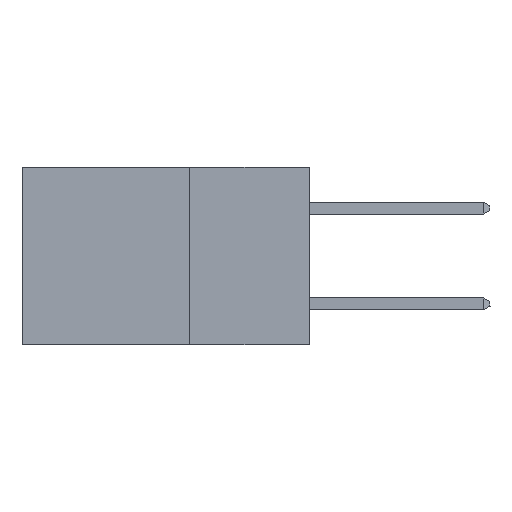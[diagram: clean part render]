
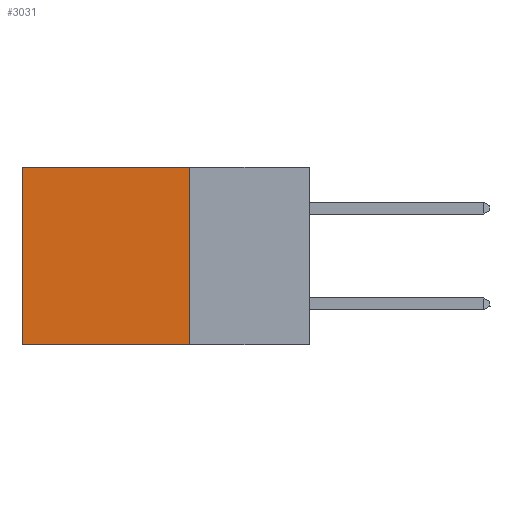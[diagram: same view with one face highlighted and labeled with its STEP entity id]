
A CAD part, left-side view. The second image highlights one B-rep face of the part: STEP entity #3031.
In plain terms, the highlighted planar face has unit normal (-1, 0, 0).
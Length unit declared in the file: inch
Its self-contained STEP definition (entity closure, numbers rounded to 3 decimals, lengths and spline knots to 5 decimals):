
#345 = CARTESIAN_POINT ( 'NONE',  ( 0.2875, 0.25, 0. ) ) ;
#1156 = LINE ( 'NONE', #7265, #6009 ) ;
#1166 = VERTEX_POINT ( 'NONE', #6011 ) ;
#2378 = EDGE_CURVE ( 'NONE', #4305, #11347, #8157, .T. ) ;
#2562 = DIRECTION ( 'NONE',  ( 0., 0., -1. ) ) ;
#2623 = DIRECTION ( 'NONE',  ( 0., 1., 0. ) ) ;
#3031 = ADVANCED_FACE ( 'NONE', ( #11648 ), #6166, .F. ) ;
#3062 = ORIENTED_EDGE ( 'NONE', *, *, #2378, .T. ) ;
#3473 = CARTESIAN_POINT ( 'NONE',  ( 0.2875, 0.6, 0. ) ) ;
#3882 = EDGE_LOOP ( 'NONE', ( #3062, #8256, #6002, #8533 ) ) ;
#4157 = CARTESIAN_POINT ( 'NONE',  ( 0.2875, 0.6, -0.37 ) ) ;
#4305 = VERTEX_POINT ( 'NONE', #3473 ) ;
#5493 = CARTESIAN_POINT ( 'NONE',  ( 0.2875, 0.25, 0. ) ) ;
#6002 = ORIENTED_EDGE ( 'NONE', *, *, #10012, .F. ) ;
#6009 = VECTOR ( 'NONE', #10042, 39.37008 ) ;
#6011 = CARTESIAN_POINT ( 'NONE',  ( 0.2875, 0.25, 0. ) ) ;
#6166 = PLANE ( 'NONE',  #11304 ) ;
#6210 = DIRECTION ( 'NONE',  ( 0., 0., -1. ) ) ;
#7265 = CARTESIAN_POINT ( 'NONE',  ( 0.2875, 0.25, -0.37 ) ) ;
#7585 = CARTESIAN_POINT ( 'NONE',  ( 0.2875, 0.25, 0. ) ) ;
#7998 = LINE ( 'NONE', #345, #10208 ) ;
#8114 = LINE ( 'NONE', #7585, #12831 ) ;
#8157 = LINE ( 'NONE', #11780, #10348 ) ;
#8256 = ORIENTED_EDGE ( 'NONE', *, *, #11508, .F. ) ;
#8533 = ORIENTED_EDGE ( 'NONE', *, *, #11837, .T. ) ;
#10012 = EDGE_CURVE ( 'NONE', #1166, #12093, #7998, .T. ) ;
#10042 = DIRECTION ( 'NONE',  ( 0., 1., 0. ) ) ;
#10208 = VECTOR ( 'NONE', #2562, 39.37008 ) ;
#10348 = VECTOR ( 'NONE', #12187, 39.37008 ) ;
#10655 = CARTESIAN_POINT ( 'NONE',  ( 0.2875, 0.25, -0.37 ) ) ;
#11304 = AXIS2_PLACEMENT_3D ( 'NONE', #5493, #11750, #6210 ) ;
#11347 = VERTEX_POINT ( 'NONE', #4157 ) ;
#11508 = EDGE_CURVE ( 'NONE', #12093, #11347, #1156, .T. ) ;
#11648 = FACE_OUTER_BOUND ( 'NONE', #3882, .T. ) ;
#11750 = DIRECTION ( 'NONE',  ( 1., 0., 0. ) ) ;
#11780 = CARTESIAN_POINT ( 'NONE',  ( 0.2875, 0.6, 0. ) ) ;
#11837 = EDGE_CURVE ( 'NONE', #1166, #4305, #8114, .T. ) ;
#12093 = VERTEX_POINT ( 'NONE', #10655 ) ;
#12187 = DIRECTION ( 'NONE',  ( 0., 0., -1. ) ) ;
#12831 = VECTOR ( 'NONE', #2623, 39.37008 ) ;
